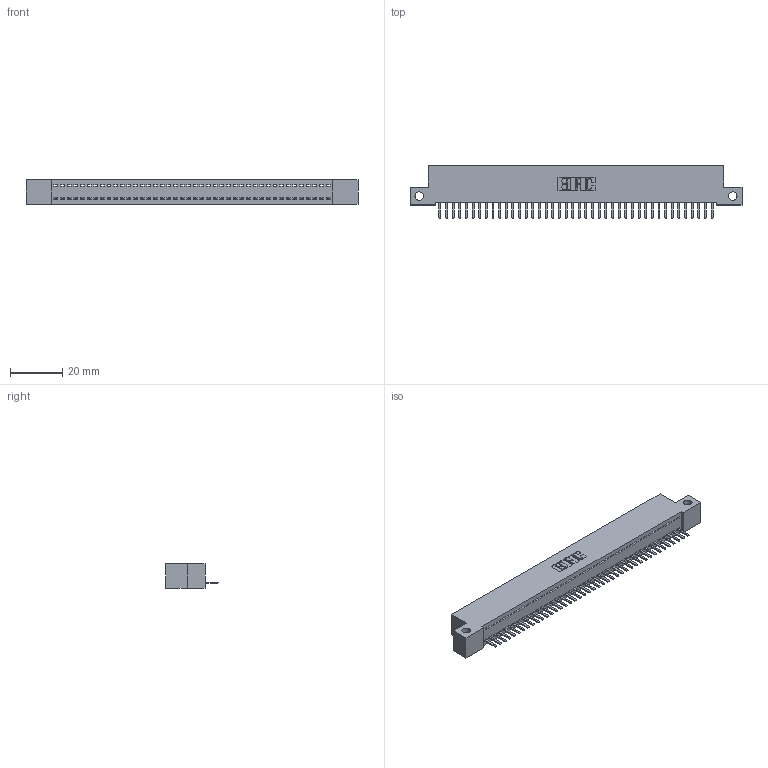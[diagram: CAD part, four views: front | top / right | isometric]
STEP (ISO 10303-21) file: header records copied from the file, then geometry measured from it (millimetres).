
FILE_DESCRIPTION (( 'STEP AP203' ), '1' );
FILE_NAME ('392-042-520-112.STEP', '2018-08-16T13:11:24', ( '' ), ( '' ), 'SwSTEP 2.0', 'SolidWorks 2016', '' );
FILE_SCHEMA (( 'CONFIG_CONTROL_DESIGN' ));
Length unit declared in the file: inch
Products named in the file (3): 342 Part_Side Mount; 345-292-001_345-293-120; 392-042-520-112
Assembly tree (43 placements, depth 2):
  392-042-520-112
    342 Part_Side Mount
    345-292-001_345-293-120  x42
Bounding box: 127 x 20.02 x 9.4 mm (x, y, z)
Volume: 10940.6 mm3; surface area: 15516.3 mm2
Topology: 43 solids, 43 shells, 2714 faces, 8027 edges, 5238 vertices
Faces by surface type: plane 1914, cylinder 800
Entity records: 25661 total; most frequent: CARTESIAN_POINT 4444, ORIENTED_EDGE 4410, DIRECTION 3737, EDGE_CURVE 2205, LINE 2073, VECTOR 2073, VERTEX_POINT 1466, AXIS2_PLACEMENT_3D 832
